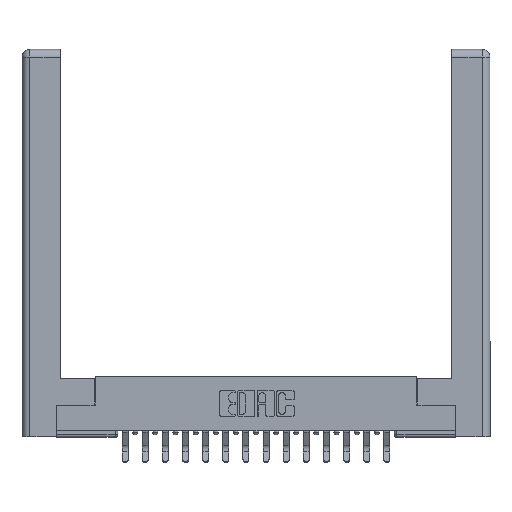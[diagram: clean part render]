
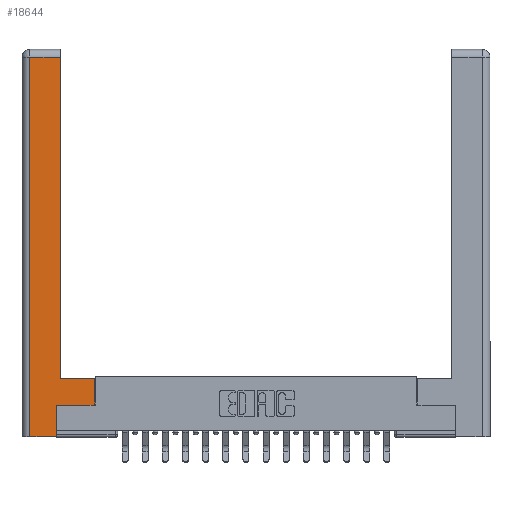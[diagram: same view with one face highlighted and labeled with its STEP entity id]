
A CAD part, top view. The second image highlights one B-rep face of the part: STEP entity #18644.
In plain terms, the highlighted planar face has unit normal (0, 0, 1).
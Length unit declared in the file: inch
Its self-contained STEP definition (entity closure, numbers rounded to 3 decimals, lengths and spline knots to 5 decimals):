
#180 = CARTESIAN_POINT ( 'NONE',  ( 0.0615, 0., 0. ) ) ;
#1229 = CARTESIAN_POINT ( 'NONE',  ( 0.0615, 2.94, 0. ) ) ;
#1317 = LINE ( 'NONE', #6980, #5360 ) ;
#1426 = VECTOR ( 'NONE', #15513, 39.37008 ) ;
#1715 = CARTESIAN_POINT ( 'NONE',  ( 0.295, 0.45, 0. ) ) ;
#1737 = VERTEX_POINT ( 'NONE', #5028 ) ;
#1971 = CARTESIAN_POINT ( 'NONE',  ( 0.295, 3., 0. ) ) ;
#2208 = VERTEX_POINT ( 'NONE', #13515 ) ;
#2299 = VECTOR ( 'NONE', #11992, 39.37008 ) ;
#2375 = LINE ( 'NONE', #2758, #1426 ) ;
#2578 = ORIENTED_EDGE ( 'NONE', *, *, #2869, .T. ) ;
#2639 = VECTOR ( 'NONE', #5222, 39.37008 ) ;
#2758 = CARTESIAN_POINT ( 'NONE',  ( 0.295, 0.45, 0. ) ) ;
#2869 = EDGE_CURVE ( 'NONE', #8338, #15061, #12426, .T. ) ;
#3464 = PLANE ( 'NONE',  #10904 ) ;
#3501 = DIRECTION ( 'NONE',  ( 0., 1., 0. ) ) ;
#5028 = CARTESIAN_POINT ( 'NONE',  ( 0.295, 2.94, 0. ) ) ;
#5043 = LINE ( 'NONE', #7899, #17795 ) ;
#5222 = DIRECTION ( 'NONE',  ( 1., 0., 0. ) ) ;
#5360 = VECTOR ( 'NONE', #8505, 39.37008 ) ;
#5656 = VECTOR ( 'NONE', #3501, 39.37008 ) ;
#5892 = LINE ( 'NONE', #7028, #13065 ) ;
#5969 = VERTEX_POINT ( 'NONE', #1715 ) ;
#6616 = ORIENTED_EDGE ( 'NONE', *, *, #15189, .T. ) ;
#6980 = CARTESIAN_POINT ( 'NONE',  ( 0.565, 0.245, 0. ) ) ;
#7028 = CARTESIAN_POINT ( 'NONE',  ( 0.0615, 2.94, 0. ) ) ;
#7249 = EDGE_CURVE ( 'NONE', #15061, #8104, #12997, .T. ) ;
#7808 = FACE_OUTER_BOUND ( 'NONE', #7893, .T. ) ;
#7893 = EDGE_LOOP ( 'NONE', ( #8729, #12960, #8949, #2578, #13889, #12044, #6616, #15292 ) ) ;
#7899 = CARTESIAN_POINT ( 'NONE',  ( 0.0615, 0., 0. ) ) ;
#7901 = DIRECTION ( 'NONE',  ( -1., 0., 0. ) ) ;
#8031 = CARTESIAN_POINT ( 'NONE',  ( 0.565, 0.45, 0. ) ) ;
#8104 = VERTEX_POINT ( 'NONE', #8218 ) ;
#8218 = CARTESIAN_POINT ( 'NONE',  ( 0.265, 0.245, 0. ) ) ;
#8338 = VERTEX_POINT ( 'NONE', #180 ) ;
#8505 = DIRECTION ( 'NONE',  ( 1., 0., 0. ) ) ;
#8588 = EDGE_CURVE ( 'NONE', #1737, #9312, #5892, .T. ) ;
#8729 = ORIENTED_EDGE ( 'NONE', *, *, #13870, .T. ) ;
#8949 = ORIENTED_EDGE ( 'NONE', *, *, #17377, .T. ) ;
#9312 = VERTEX_POINT ( 'NONE', #1229 ) ;
#9336 = DIRECTION ( 'NONE',  ( 0., 0., -1. ) ) ;
#9372 = LINE ( 'NONE', #8031, #5656 ) ;
#9596 = VERTEX_POINT ( 'NONE', #13617 ) ;
#10904 = AXIS2_PLACEMENT_3D ( 'NONE', #17740, #9336, #7901 ) ;
#11992 = DIRECTION ( 'NONE',  ( 0., 1., 0. ) ) ;
#12044 = ORIENTED_EDGE ( 'NONE', *, *, #15346, .T. ) ;
#12426 = LINE ( 'NONE', #18184, #2639 ) ;
#12806 = DIRECTION ( 'NONE',  ( 0., 1., 0. ) ) ;
#12960 = ORIENTED_EDGE ( 'NONE', *, *, #8588, .T. ) ;
#12997 = LINE ( 'NONE', #18637, #16472 ) ;
#13065 = VECTOR ( 'NONE', #17338, 39.37008 ) ;
#13515 = CARTESIAN_POINT ( 'NONE',  ( 0.565, 0.45, 0. ) ) ;
#13617 = CARTESIAN_POINT ( 'NONE',  ( 0.565, 0.245, 0. ) ) ;
#13870 = EDGE_CURVE ( 'NONE', #5969, #1737, #14937, .T. ) ;
#13889 = ORIENTED_EDGE ( 'NONE', *, *, #7249, .T. ) ;
#14920 = EDGE_CURVE ( 'NONE', #2208, #5969, #2375, .T. ) ;
#14937 = LINE ( 'NONE', #1971, #2299 ) ;
#15061 = VERTEX_POINT ( 'NONE', #17315 ) ;
#15189 = EDGE_CURVE ( 'NONE', #9596, #2208, #9372, .T. ) ;
#15292 = ORIENTED_EDGE ( 'NONE', *, *, #14920, .T. ) ;
#15346 = EDGE_CURVE ( 'NONE', #8104, #9596, #1317, .T. ) ;
#15513 = DIRECTION ( 'NONE',  ( -1., 0., 0. ) ) ;
#16472 = VECTOR ( 'NONE', #12806, 39.37008 ) ;
#17315 = CARTESIAN_POINT ( 'NONE',  ( 0.265, 0., 0. ) ) ;
#17338 = DIRECTION ( 'NONE',  ( -1., 0., 0. ) ) ;
#17377 = EDGE_CURVE ( 'NONE', #9312, #8338, #5043, .T. ) ;
#17740 = CARTESIAN_POINT ( 'NONE',  ( 0., 0., 0. ) ) ;
#17795 = VECTOR ( 'NONE', #18014, 39.37008 ) ;
#18014 = DIRECTION ( 'NONE',  ( 0., -1., 0. ) ) ;
#18184 = CARTESIAN_POINT ( 'NONE',  ( 0.265, 0., 0. ) ) ;
#18637 = CARTESIAN_POINT ( 'NONE',  ( 0.265, 0.245, 0. ) ) ;
#18644 = ADVANCED_FACE ( 'NONE', ( #7808 ), #3464, .F. ) ;
